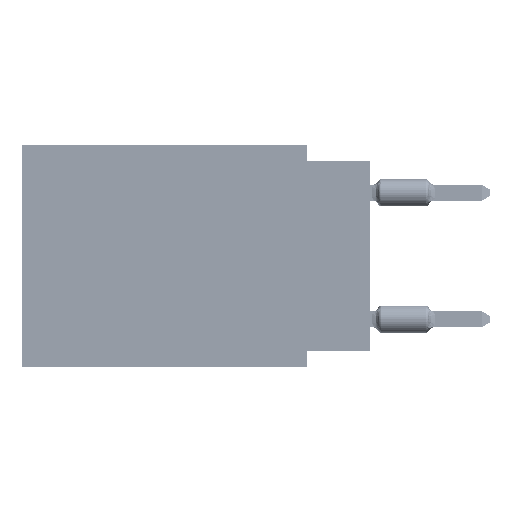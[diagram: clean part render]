
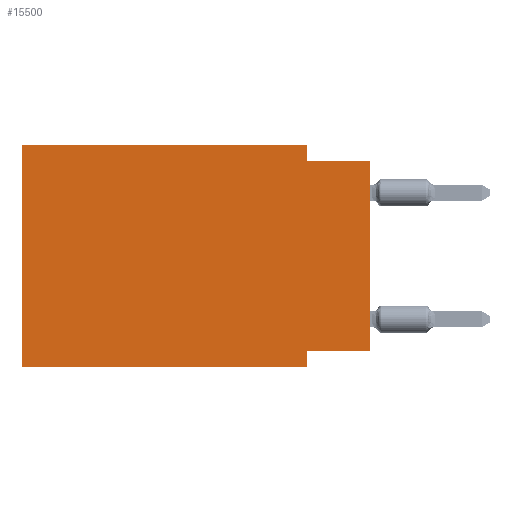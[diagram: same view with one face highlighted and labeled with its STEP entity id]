
A CAD part, left-side view. The second image highlights one B-rep face of the part: STEP entity #15500.
In plain terms, the highlighted planar face has unit normal (-1, 0, 0).
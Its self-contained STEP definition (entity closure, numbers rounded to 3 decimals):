
#1400 = VERTEX_POINT ( 'NONE', #15678 ) ;
#3035 = LINE ( 'NONE', #59796, #26502 ) ;
#3133 = CARTESIAN_POINT ( 'NONE',  ( 0., 13.97, 0. ) ) ;
#4138 = DIRECTION ( 'NONE',  ( 0., 0., 1. ) ) ;
#4469 = LINE ( 'NONE', #3133, #38792 ) ;
#5155 = EDGE_CURVE ( 'NONE', #63027, #23404, #34561, .T. ) ;
#8314 = CARTESIAN_POINT ( 'NONE',  ( 0., 13.97, -8.89 ) ) ;
#12062 = LINE ( 'NONE', #16845, #62818 ) ;
#13373 = EDGE_CURVE ( 'NONE', #38801, #67525, #12062, .T. ) ;
#13526 = CARTESIAN_POINT ( 'NONE',  ( 0., 0., -0.635 ) ) ;
#13695 = FACE_OUTER_BOUND ( 'NONE', #51235, .T. ) ;
#14147 = VERTEX_POINT ( 'NONE', #64125 ) ;
#14709 = PLANE ( 'NONE',  #48818 ) ;
#15500 = ADVANCED_FACE ( 'NONE', ( #13695 ), #14709, .F. ) ;
#15678 = CARTESIAN_POINT ( 'NONE',  ( 0., 2.54, -8.89 ) ) ;
#16845 = CARTESIAN_POINT ( 'NONE',  ( 0., 2.54, 0. ) ) ;
#18820 = DIRECTION ( 'NONE',  ( 0., 0., -1. ) ) ;
#19855 = DIRECTION ( 'NONE',  ( 0., 0., 1. ) ) ;
#20880 = DIRECTION ( 'NONE',  ( 0., -1., 0. ) ) ;
#21224 = DIRECTION ( 'NONE',  ( 0., 0., -1. ) ) ;
#23404 = VERTEX_POINT ( 'NONE', #13526 ) ;
#24146 = ORIENTED_EDGE ( 'NONE', *, *, #13373, .F. ) ;
#24591 = EDGE_CURVE ( 'NONE', #14147, #38801, #3035, .T. ) ;
#24975 = DIRECTION ( 'NONE',  ( 1., 0., 0. ) ) ;
#26502 = VECTOR ( 'NONE', #44395, 1000. ) ;
#27710 = LINE ( 'NONE', #28059, #53833 ) ;
#28059 = CARTESIAN_POINT ( 'NONE',  ( 0., 0., -8.255 ) ) ;
#28214 = ORIENTED_EDGE ( 'NONE', *, *, #64787, .F. ) ;
#28607 = CARTESIAN_POINT ( 'NONE',  ( 0., 2.54, -0.635 ) ) ;
#29173 = DIRECTION ( 'NONE',  ( 0., -1., 0. ) ) ;
#31797 = CARTESIAN_POINT ( 'NONE',  ( 0., 0., -0.635 ) ) ;
#33609 = ORIENTED_EDGE ( 'NONE', *, *, #24591, .F. ) ;
#34561 = LINE ( 'NONE', #67034, #45485 ) ;
#36387 = EDGE_CURVE ( 'NONE', #63139, #1400, #66733, .T. ) ;
#36658 = EDGE_CURVE ( 'NONE', #63027, #63139, #27710, .T. ) ;
#38422 = CARTESIAN_POINT ( 'NONE',  ( 0., 2.54, -8.255 ) ) ;
#38792 = VECTOR ( 'NONE', #4138, 1000. ) ;
#38801 = VERTEX_POINT ( 'NONE', #61625 ) ;
#40197 = ORIENTED_EDGE ( 'NONE', *, *, #5155, .T. ) ;
#40722 = CARTESIAN_POINT ( 'NONE',  ( 0., 13.97, -8.89 ) ) ;
#41487 = ORIENTED_EDGE ( 'NONE', *, *, #66056, .F. ) ;
#42024 = ORIENTED_EDGE ( 'NONE', *, *, #49740, .T. ) ;
#42400 = LINE ( 'NONE', #31797, #44410 ) ;
#44395 = DIRECTION ( 'NONE',  ( 0., -1., 0. ) ) ;
#44410 = VECTOR ( 'NONE', #20880, 1000. ) ;
#45485 = VECTOR ( 'NONE', #19855, 1000. ) ;
#48818 = AXIS2_PLACEMENT_3D ( 'NONE', #66683, #24975, #18820 ) ;
#49740 = EDGE_CURVE ( 'NONE', #53942, #1400, #64755, .T. ) ;
#50718 = ORIENTED_EDGE ( 'NONE', *, *, #36658, .F. ) ;
#51235 = EDGE_LOOP ( 'NONE', ( #40197, #41487, #24146, #33609, #28214, #42024, #52233, #50718 ) ) ;
#52233 = ORIENTED_EDGE ( 'NONE', *, *, #36387, .F. ) ;
#53833 = VECTOR ( 'NONE', #64306, 1000. ) ;
#53942 = VERTEX_POINT ( 'NONE', #40722 ) ;
#56470 = CARTESIAN_POINT ( 'NONE',  ( 0., 2.54, -8.89 ) ) ;
#57925 = CARTESIAN_POINT ( 'NONE',  ( 0., 0., -8.255 ) ) ;
#58223 = VECTOR ( 'NONE', #21224, 1000. ) ;
#59796 = CARTESIAN_POINT ( 'NONE',  ( 0., 13.97, 0. ) ) ;
#61625 = CARTESIAN_POINT ( 'NONE',  ( 0., 2.54, 0. ) ) ;
#62818 = VECTOR ( 'NONE', #64022, 1000. ) ;
#63027 = VERTEX_POINT ( 'NONE', #57925 ) ;
#63139 = VERTEX_POINT ( 'NONE', #38422 ) ;
#64022 = DIRECTION ( 'NONE',  ( 0., 0., -1. ) ) ;
#64125 = CARTESIAN_POINT ( 'NONE',  ( 0., 13.97, 0. ) ) ;
#64306 = DIRECTION ( 'NONE',  ( 0., 1., 0. ) ) ;
#64755 = LINE ( 'NONE', #8314, #65281 ) ;
#64787 = EDGE_CURVE ( 'NONE', #53942, #14147, #4469, .T. ) ;
#65281 = VECTOR ( 'NONE', #29173, 1000. ) ;
#66056 = EDGE_CURVE ( 'NONE', #67525, #23404, #42400, .T. ) ;
#66683 = CARTESIAN_POINT ( 'NONE',  ( 0., 13.97, 0. ) ) ;
#66733 = LINE ( 'NONE', #56470, #58223 ) ;
#67034 = CARTESIAN_POINT ( 'NONE',  ( 0., 0., 0. ) ) ;
#67525 = VERTEX_POINT ( 'NONE', #28607 ) ;
